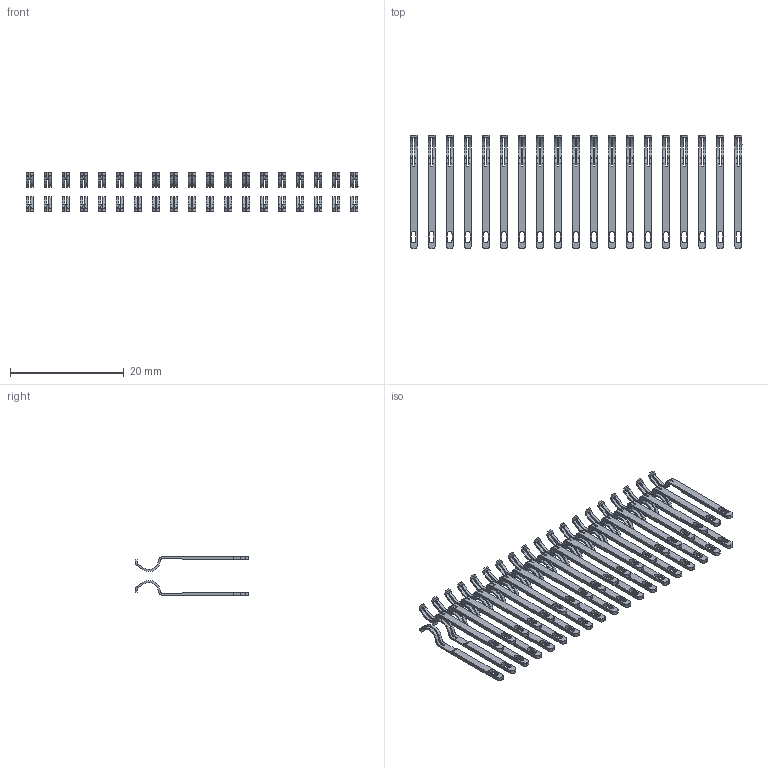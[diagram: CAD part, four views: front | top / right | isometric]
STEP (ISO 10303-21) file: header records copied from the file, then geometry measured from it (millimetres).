
FILE_DESCRIPTION (( 'STEP AP203' ), '1' );
FILE_NAME ('346-038-500-802.STEP', '2018-08-24T04:19:58', ( '' ), ( '' ), 'SwSTEP 2.0', 'SolidWorks 2016', '' );
FILE_SCHEMA (( 'CONFIG_CONTROL_DESIGN' ));
Length unit declared in the file: inch
Products named in the file (3): 346 Part_0.170 Offset - 0.128 Dia; 345-292-001_345-293-100; 346-038-500-802
Assembly tree (39 placements, depth 2):
  346-038-500-802
    346 Part_0.170 Offset - 0.128 Dia
    345-292-001_345-293-100  x38
Bounding box: 58.42 x 19.94 x 6.99 mm (x, y, z)
Volume: 458 mm3; surface area: 2999.4 mm2
Topology: 38 solids, 38 shells, 1596 faces, 4788 edges, 3192 vertices
Faces by surface type: plane 912, cylinder 684
Entity records: 15561 total; most frequent: CARTESIAN_POINT 2596, ORIENTED_EDGE 2530, DIRECTION 2341, EDGE_CURVE 1265, LINE 1053, VECTOR 1053, VERTEX_POINT 842, AXIS2_PLACEMENT_3D 644
